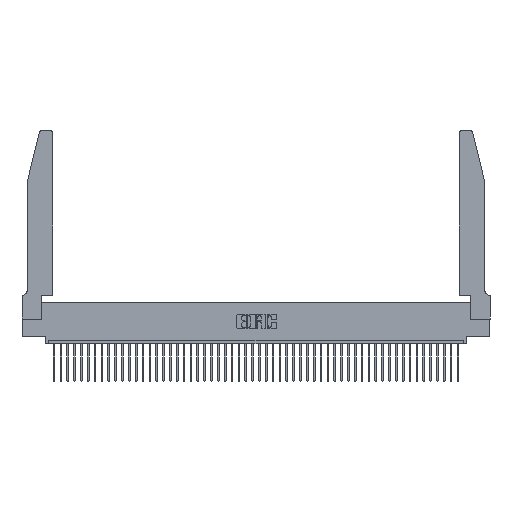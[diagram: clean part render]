
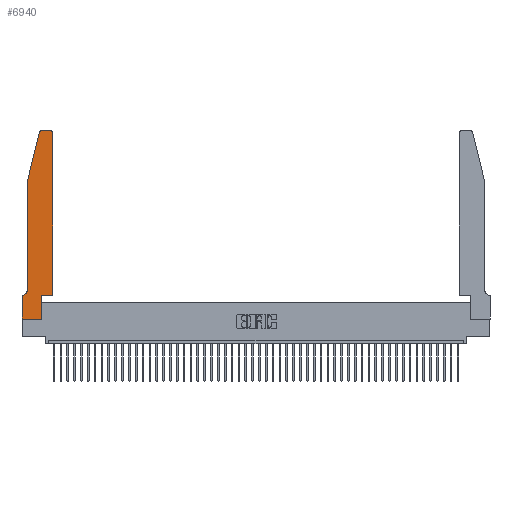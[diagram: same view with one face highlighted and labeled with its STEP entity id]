
A CAD part, top view. The second image highlights one B-rep face of the part: STEP entity #6940.
In plain terms, the highlighted planar face has unit normal (0, 0, 1).
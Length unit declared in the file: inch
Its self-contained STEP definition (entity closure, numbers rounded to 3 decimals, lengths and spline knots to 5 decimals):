
#1084 = VERTEX_POINT ( 'NONE', #46594 ) ;
#1618 = VERTEX_POINT ( 'NONE', #17389 ) ;
#3429 = CARTESIAN_POINT ( 'NONE',  ( 0.4505, 2.72, 0.37 ) ) ;
#3597 = VECTOR ( 'NONE', #10028, 39.37008 ) ;
#3795 = EDGE_CURVE ( 'NONE', #34796, #5540, #15981, .T. ) ;
#3850 = CIRCLE ( 'NONE', #10141, 0.03 ) ;
#4067 = DIRECTION ( 'NONE',  ( 1., 0., 0. ) ) ;
#4187 = ORIENTED_EDGE ( 'NONE', *, *, #3795, .T. ) ;
#4228 = CARTESIAN_POINT ( 'NONE',  ( 0.284, 2.72, 0.37 ) ) ;
#4382 = DIRECTION ( 'NONE',  ( 0., 0., 1. ) ) ;
#4658 = CARTESIAN_POINT ( 'NONE',  ( 0.4505, 0.35, 0.37 ) ) ;
#4727 = CARTESIAN_POINT ( 'NONE',  ( 0.4205, 2.75, 0.37 ) ) ;
#5289 = EDGE_CURVE ( 'NONE', #44261, #36362, #8891, .T. ) ;
#5540 = VERTEX_POINT ( 'NONE', #25698 ) ;
#5623 = DIRECTION ( 'NONE',  ( 0., 0., 1. ) ) ;
#5865 = FACE_OUTER_BOUND ( 'NONE', #27821, .T. ) ;
#5906 = VECTOR ( 'NONE', #11815, 39.37008 ) ;
#6188 = VECTOR ( 'NONE', #25460, 39.37008 ) ;
#6262 = DIRECTION ( 'NONE',  ( 0., 0., -1. ) ) ;
#6829 = EDGE_CURVE ( 'NONE', #46425, #1618, #25409, .T. ) ;
#6940 = ADVANCED_FACE ( 'NONE', ( #5865 ), #45970, .T. ) ;
#6952 = CARTESIAN_POINT ( 'NONE',  ( 0., 0., 0.37 ) ) ;
#7038 = DIRECTION ( 'NONE',  ( 0., -1., 0. ) ) ;
#8549 = ORIENTED_EDGE ( 'NONE', *, *, #23430, .T. ) ;
#8891 = CIRCLE ( 'NONE', #28081, 0.07 ) ;
#9475 = DIRECTION ( 'NONE',  ( 1., 0., 0. ) ) ;
#9652 = EDGE_CURVE ( 'NONE', #34534, #26549, #26582, .T. ) ;
#10028 = DIRECTION ( 'NONE',  ( -1., 0., 0. ) ) ;
#10141 = AXIS2_PLACEMENT_3D ( 'NONE', #4228, #4382, #4067 ) ;
#11210 = CARTESIAN_POINT ( 'NONE',  ( 0.0755, 0.35, 0.37 ) ) ;
#11214 = CARTESIAN_POINT ( 'NONE',  ( 0.4205, 2.72, 0.37 ) ) ;
#11267 = EDGE_CURVE ( 'NONE', #26549, #46425, #38522, .T. ) ;
#11728 = ORIENTED_EDGE ( 'NONE', *, *, #6829, .T. ) ;
#11815 = DIRECTION ( 'NONE',  ( 1., 0., 0. ) ) ;
#12358 = CARTESIAN_POINT ( 'NONE',  ( 0.2865, 0.35, 0.37 ) ) ;
#12544 = CARTESIAN_POINT ( 'NONE',  ( 0., 0.35, 0.37 ) ) ;
#12774 = VECTOR ( 'NONE', #26672, 39.37008 ) ;
#12796 = CARTESIAN_POINT ( 'NONE',  ( 0.0755, 0.42, 0.37 ) ) ;
#13792 = DIRECTION ( 'NONE',  ( 0., 1., 0. ) ) ;
#15724 = EDGE_CURVE ( 'NONE', #30438, #28760, #27723, .T. ) ;
#15981 = LINE ( 'NONE', #17612, #6188 ) ;
#16190 = ORIENTED_EDGE ( 'NONE', *, *, #5289, .T. ) ;
#17389 = CARTESIAN_POINT ( 'NONE',  ( 0.4505, 0.35, 0.37 ) ) ;
#17612 = CARTESIAN_POINT ( 'NONE',  ( 0.0755, 2., 0.37 ) ) ;
#18256 = EDGE_CURVE ( 'NONE', #28760, #34796, #3850, .T. ) ;
#18626 = DIRECTION ( 'NONE',  ( 1., 0., 0. ) ) ;
#18696 = DIRECTION ( 'NONE',  ( 0., -1., 0. ) ) ;
#18800 = CIRCLE ( 'NONE', #27493, 0.03 ) ;
#19858 = EDGE_CURVE ( 'NONE', #1618, #33473, #26165, .T. ) ;
#20451 = CARTESIAN_POINT ( 'NONE',  ( 0.0055, 0.35, 0.37 ) ) ;
#20549 = ORIENTED_EDGE ( 'NONE', *, *, #43993, .T. ) ;
#22714 = ORIENTED_EDGE ( 'NONE', *, *, #24561, .T. ) ;
#23430 = EDGE_CURVE ( 'NONE', #33473, #30438, #18800, .T. ) ;
#24045 = ORIENTED_EDGE ( 'NONE', *, *, #9652, .T. ) ;
#24561 = EDGE_CURVE ( 'NONE', #36362, #1084, #34154, .T. ) ;
#24595 = ORIENTED_EDGE ( 'NONE', *, *, #15724, .T. ) ;
#24756 = CARTESIAN_POINT ( 'NONE',  ( 0., 0., 0.37 ) ) ;
#25409 = LINE ( 'NONE', #4658, #12774 ) ;
#25460 = DIRECTION ( 'NONE',  ( -0.239, -0.971, 0. ) ) ;
#25698 = CARTESIAN_POINT ( 'NONE',  ( 0.0755, 2., 0.37 ) ) ;
#26165 = LINE ( 'NONE', #31931, #28488 ) ;
#26549 = VERTEX_POINT ( 'NONE', #34771 ) ;
#26582 = LINE ( 'NONE', #24756, #5906 ) ;
#26672 = DIRECTION ( 'NONE',  ( 1., 0., 0. ) ) ;
#27493 = AXIS2_PLACEMENT_3D ( 'NONE', #11214, #40653, #18626 ) ;
#27665 = LINE ( 'NONE', #43746, #35749 ) ;
#27723 = LINE ( 'NONE', #42841, #3597 ) ;
#27821 = EDGE_LOOP ( 'NONE', ( #24595, #32470, #4187, #20549, #16190, #22714, #28693, #24045, #34629, #11728, #38464, #8549 ) ) ;
#28081 = AXIS2_PLACEMENT_3D ( 'NONE', #34884, #6262, #47085 ) ;
#28488 = VECTOR ( 'NONE', #13792, 39.37008 ) ;
#28693 = ORIENTED_EDGE ( 'NONE', *, *, #40114, .T. ) ;
#28735 = VECTOR ( 'NONE', #36075, 39.37008 ) ;
#28760 = VERTEX_POINT ( 'NONE', #46089 ) ;
#30438 = VERTEX_POINT ( 'NONE', #4727 ) ;
#31871 = CARTESIAN_POINT ( 'NONE',  ( 0., 0., 0.37 ) ) ;
#31931 = CARTESIAN_POINT ( 'NONE',  ( 0.4505, 0.35, 0.37 ) ) ;
#32470 = ORIENTED_EDGE ( 'NONE', *, *, #18256, .T. ) ;
#33473 = VERTEX_POINT ( 'NONE', #3429 ) ;
#33560 = DIRECTION ( 'NONE',  ( -1., 0., 0. ) ) ;
#34154 = LINE ( 'NONE', #11210, #36487 ) ;
#34534 = VERTEX_POINT ( 'NONE', #31871 ) ;
#34629 = ORIENTED_EDGE ( 'NONE', *, *, #11267, .T. ) ;
#34771 = CARTESIAN_POINT ( 'NONE',  ( 0.2865, 0., 0.37 ) ) ;
#34796 = VERTEX_POINT ( 'NONE', #40740 ) ;
#34884 = CARTESIAN_POINT ( 'NONE',  ( 0.0055, 0.42, 0.37 ) ) ;
#35749 = VECTOR ( 'NONE', #7038, 39.37008 ) ;
#36075 = DIRECTION ( 'NONE',  ( 0., 1., 0. ) ) ;
#36362 = VERTEX_POINT ( 'NONE', #20451 ) ;
#36487 = VECTOR ( 'NONE', #33560, 39.37008 ) ;
#38370 = VECTOR ( 'NONE', #18696, 39.37008 ) ;
#38464 = ORIENTED_EDGE ( 'NONE', *, *, #19858, .T. ) ;
#38522 = LINE ( 'NONE', #42513, #28735 ) ;
#39921 = AXIS2_PLACEMENT_3D ( 'NONE', #12544, #5623, #9475 ) ;
#40114 = EDGE_CURVE ( 'NONE', #1084, #34534, #47007, .T. ) ;
#40653 = DIRECTION ( 'NONE',  ( 0., 0., 1. ) ) ;
#40740 = CARTESIAN_POINT ( 'NONE',  ( 0.25487, 2.72718, 0.37 ) ) ;
#42513 = CARTESIAN_POINT ( 'NONE',  ( 0.2865, 0.35, 0.37 ) ) ;
#42841 = CARTESIAN_POINT ( 'NONE',  ( 0.2605, 2.75, 0.37 ) ) ;
#43746 = CARTESIAN_POINT ( 'NONE',  ( 0.0755, 2., 0.37 ) ) ;
#43993 = EDGE_CURVE ( 'NONE', #5540, #44261, #27665, .T. ) ;
#44261 = VERTEX_POINT ( 'NONE', #12796 ) ;
#45970 = PLANE ( 'NONE',  #39921 ) ;
#46089 = CARTESIAN_POINT ( 'NONE',  ( 0.284, 2.75, 0.37 ) ) ;
#46425 = VERTEX_POINT ( 'NONE', #12358 ) ;
#46594 = CARTESIAN_POINT ( 'NONE',  ( 0., 0.35, 0.37 ) ) ;
#47007 = LINE ( 'NONE', #6952, #38370 ) ;
#47085 = DIRECTION ( 'NONE',  ( -1., 0., 0. ) ) ;
